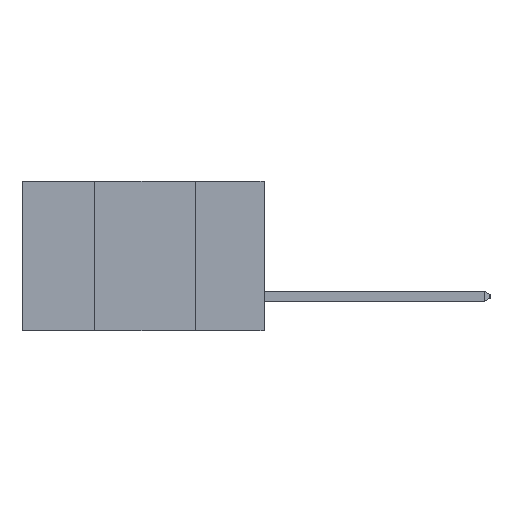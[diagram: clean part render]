
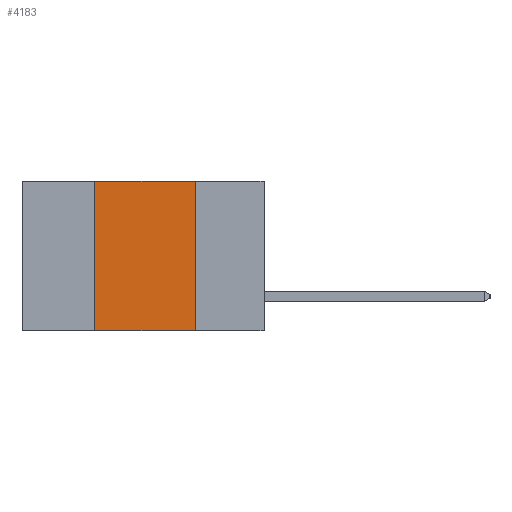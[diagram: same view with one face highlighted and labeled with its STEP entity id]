
A CAD part, left-side view. The second image highlights one B-rep face of the part: STEP entity #4183.
In plain terms, the highlighted planar face has unit normal (-1, 0, 0).
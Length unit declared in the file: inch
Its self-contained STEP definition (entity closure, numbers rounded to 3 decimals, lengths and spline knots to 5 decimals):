
#11 = ORIENTED_EDGE ( 'NONE', *, *, #9987, .F. ) ;
#140 = CARTESIAN_POINT ( 'NONE',  ( 0., 0.6, -0.37 ) ) ;
#202 = AXIS2_PLACEMENT_3D ( 'NONE', #8037, #257, #6380 ) ;
#257 = DIRECTION ( 'NONE',  ( 1., 0., 0. ) ) ;
#1041 = VECTOR ( 'NONE', #6959, 39.37008 ) ;
#1284 = DIRECTION ( 'NONE',  ( 0., -1., 0. ) ) ;
#1326 = LINE ( 'NONE', #1799, #1041 ) ;
#1522 = DIRECTION ( 'NONE',  ( 0., 0., 1. ) ) ;
#1627 = ORIENTED_EDGE ( 'NONE', *, *, #8303, .F. ) ;
#1799 = CARTESIAN_POINT ( 'NONE',  ( 0., 0.17, -0.37 ) ) ;
#2041 = CARTESIAN_POINT ( 'NONE',  ( 0., 0.42, -0.37 ) ) ;
#2063 = VERTEX_POINT ( 'NONE', #7757 ) ;
#2134 = CARTESIAN_POINT ( 'NONE',  ( 0., 0.6, 0. ) ) ;
#3122 = ORIENTED_EDGE ( 'NONE', *, *, #6615, .T. ) ;
#3156 = CARTESIAN_POINT ( 'NONE',  ( 0., 0.42, 0. ) ) ;
#3169 = VECTOR ( 'NONE', #1284, 39.37008 ) ;
#3254 = EDGE_LOOP ( 'NONE', ( #11, #1627, #7948, #3122 ) ) ;
#3768 = FACE_OUTER_BOUND ( 'NONE', #3254, .T. ) ;
#4183 = ADVANCED_FACE ( 'NONE', ( #3768 ), #5513, .F. ) ;
#4959 = CARTESIAN_POINT ( 'NONE',  ( 0., 0.42, -0.37 ) ) ;
#5425 = VERTEX_POINT ( 'NONE', #2041 ) ;
#5513 = PLANE ( 'NONE',  #202 ) ;
#5614 = VECTOR ( 'NONE', #1522, 39.37008 ) ;
#5890 = LINE ( 'NONE', #4959, #5614 ) ;
#6380 = DIRECTION ( 'NONE',  ( 0., 0., -1. ) ) ;
#6615 = EDGE_CURVE ( 'NONE', #5425, #2063, #6951, .T. ) ;
#6697 = VECTOR ( 'NONE', #7923, 39.37008 ) ;
#6951 = LINE ( 'NONE', #140, #6697 ) ;
#6959 = DIRECTION ( 'NONE',  ( 0., 0., -1. ) ) ;
#7168 = EDGE_CURVE ( 'NONE', #5425, #9597, #5890, .T. ) ;
#7757 = CARTESIAN_POINT ( 'NONE',  ( 0., 0.17, -0.37 ) ) ;
#7923 = DIRECTION ( 'NONE',  ( 0., -1., 0. ) ) ;
#7948 = ORIENTED_EDGE ( 'NONE', *, *, #7168, .F. ) ;
#7982 = LINE ( 'NONE', #2134, #3169 ) ;
#8037 = CARTESIAN_POINT ( 'NONE',  ( 0., 0.6, 0. ) ) ;
#8303 = EDGE_CURVE ( 'NONE', #9597, #8769, #7982, .T. ) ;
#8769 = VERTEX_POINT ( 'NONE', #10426 ) ;
#9597 = VERTEX_POINT ( 'NONE', #3156 ) ;
#9987 = EDGE_CURVE ( 'NONE', #8769, #2063, #1326, .T. ) ;
#10426 = CARTESIAN_POINT ( 'NONE',  ( 0., 0.17, 0. ) ) ;
